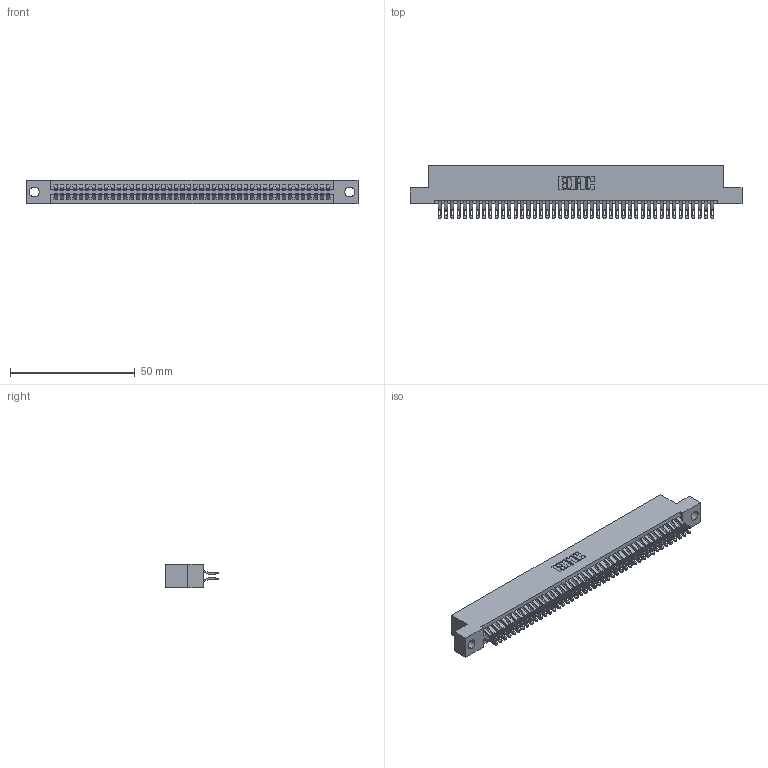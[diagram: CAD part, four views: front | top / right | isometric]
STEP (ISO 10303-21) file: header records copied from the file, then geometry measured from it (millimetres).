
FILE_DESCRIPTION (( 'STEP AP203' ), '1' );
FILE_NAME ('345-088-555-204.STEP', '2018-10-04T14:29:03', ( '' ), ( '' ), 'SwSTEP 2.0', 'SolidWorks 2016', '' );
FILE_SCHEMA (( 'CONFIG_CONTROL_DESIGN' ));
Length unit declared in the file: inch
Products named in the file (3): 345-292-001_555 Tail; 345 Part_Flush Mounting Lugs - 0.156 Dia-TH; 345-088-555-204
Assembly tree (89 placements, depth 2):
  345-088-555-204
    345 Part_Flush Mounting Lugs - 0.156 Dia-TH
    345-292-001_555 Tail  x88
Bounding box: 132.97 x 21.13 x 9.4 mm (x, y, z)
Volume: 13102.7 mm3; surface area: 20109.7 mm2
Topology: 89 solids, 89 shells, 5054 faces, 15917 edges, 10610 vertices
Faces by surface type: plane 2808, cylinder 2246
Entity records: 34583 total; most frequent: CARTESIAN_POINT 5830, ORIENTED_EDGE 5734, DIRECTION 5107, EDGE_CURVE 2867, LINE 2539, VECTOR 2539, VERTEX_POINT 1910, AXIS2_PLACEMENT_3D 1284
